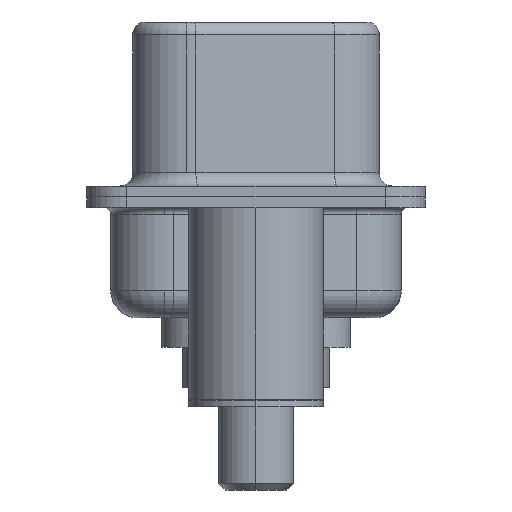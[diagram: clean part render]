
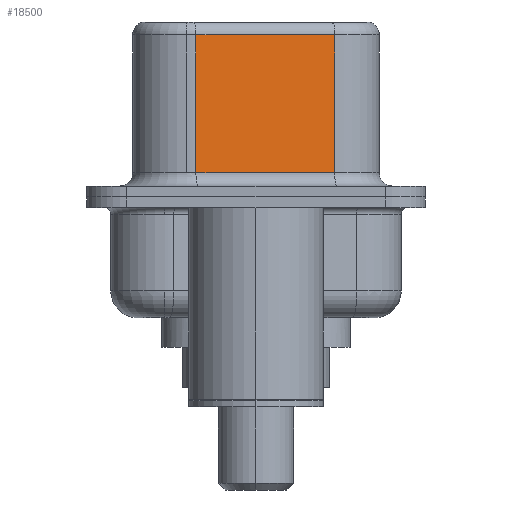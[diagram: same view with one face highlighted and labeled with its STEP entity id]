
A CAD part, left-side view. The second image highlights one B-rep face of the part: STEP entity #18500.
In plain terms, the highlighted planar face has unit normal (-0.985, -0.174, 0).
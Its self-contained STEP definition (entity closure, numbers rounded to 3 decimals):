
#49 = AXIS2_PLACEMENT_3D ( 'NONE', #16489, #7893, #17924 ) ;
#148 = CARTESIAN_POINT ( 'NONE',  ( 4.585, -2.927, 6.02 ) ) ;
#841 = VERTEX_POINT ( 'NONE', #14159 ) ;
#1641 = EDGE_CURVE ( 'NONE', #841, #6649, #3325, .T. ) ;
#2867 = ORIENTED_EDGE ( 'NONE', *, *, #10528, .T. ) ;
#3325 = LINE ( 'NONE', #11634, #6708 ) ;
#3895 = LINE ( 'NONE', #7561, #11094 ) ;
#4126 = CARTESIAN_POINT ( 'NONE',  ( 4.585, -2.927, 6.52 ) ) ;
#5348 = EDGE_LOOP ( 'NONE', ( #16629, #8641, #2867, #11966 ) ) ;
#6478 = PLANE ( 'NONE',  #49 ) ;
#6629 = VERTEX_POINT ( 'NONE', #15591 ) ;
#6649 = VERTEX_POINT ( 'NONE', #14230 ) ;
#6708 = VECTOR ( 'NONE', #12126, 1000. ) ;
#7531 = LINE ( 'NONE', #4126, #10029 ) ;
#7545 = DIRECTION ( 'NONE',  ( 0., 0., -1. ) ) ;
#7561 = CARTESIAN_POINT ( 'NONE',  ( 4.585, -2.927, 6.02 ) ) ;
#7893 = DIRECTION ( 'NONE',  ( 0.985, 0.174, 0. ) ) ;
#8641 = ORIENTED_EDGE ( 'NONE', *, *, #13581, .T. ) ;
#9750 = EDGE_CURVE ( 'NONE', #13463, #6649, #7531, .T. ) ;
#10016 = LINE ( 'NONE', #13249, #12002 ) ;
#10029 = VECTOR ( 'NONE', #11285, 1000. ) ;
#10528 = EDGE_CURVE ( 'NONE', #6629, #841, #10016, .T. ) ;
#10999 = FACE_OUTER_BOUND ( 'NONE', #5348, .T. ) ;
#11094 = VECTOR ( 'NONE', #16133, 1000. ) ;
#11285 = DIRECTION ( 'NONE',  ( 0., 0., -1. ) ) ;
#11634 = CARTESIAN_POINT ( 'NONE',  ( 4.585, -2.927, 0.9 ) ) ;
#11966 = ORIENTED_EDGE ( 'NONE', *, *, #1641, .T. ) ;
#12002 = VECTOR ( 'NONE', #7545, 1000. ) ;
#12126 = DIRECTION ( 'NONE',  ( 0.174, -0.985, 0. ) ) ;
#13249 = CARTESIAN_POINT ( 'NONE',  ( 3.675, 2.233, 6.52 ) ) ;
#13463 = VERTEX_POINT ( 'NONE', #148 ) ;
#13581 = EDGE_CURVE ( 'NONE', #13463, #6629, #3895, .T. ) ;
#14159 = CARTESIAN_POINT ( 'NONE',  ( 3.675, 2.233, 0.9 ) ) ;
#14230 = CARTESIAN_POINT ( 'NONE',  ( 4.585, -2.927, 0.9 ) ) ;
#15591 = CARTESIAN_POINT ( 'NONE',  ( 3.675, 2.233, 6.02 ) ) ;
#16133 = DIRECTION ( 'NONE',  ( -0.174, 0.985, 0. ) ) ;
#16489 = CARTESIAN_POINT ( 'NONE',  ( 4.585, -2.927, 6.52 ) ) ;
#16629 = ORIENTED_EDGE ( 'NONE', *, *, #9750, .F. ) ;
#17924 = DIRECTION ( 'NONE',  ( -0.174, 0.985, 0. ) ) ;
#18500 = ADVANCED_FACE ( 'NONE', ( #10999 ), #6478, .F. ) ;
